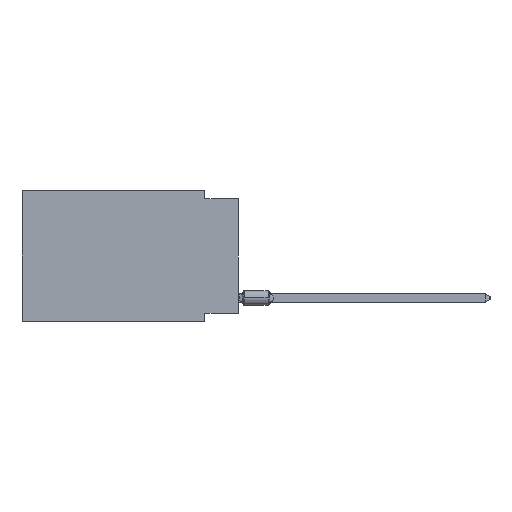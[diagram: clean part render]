
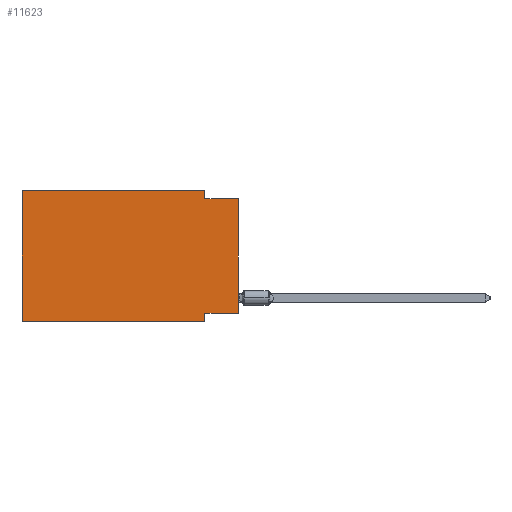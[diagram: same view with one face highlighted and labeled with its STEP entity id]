
A CAD part, left-side view. The second image highlights one B-rep face of the part: STEP entity #11623.
In plain terms, the highlighted planar face has unit normal (-1, 0, 0).
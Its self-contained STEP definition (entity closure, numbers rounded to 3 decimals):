
#2127 = ORIENTED_EDGE ( 'NONE', *, *, #6543, .F. ) ;
#3464 = DIRECTION ( 'NONE',  ( 0., 1., 0. ) ) ;
#3472 = CARTESIAN_POINT ( 'NONE',  ( 0., 16.383, 0. ) ) ;
#4175 = VERTEX_POINT ( 'NONE', #12808 ) ;
#4230 = AXIS2_PLACEMENT_3D ( 'NONE', #32441, #40569, #13186 ) ;
#4279 = CARTESIAN_POINT ( 'NONE',  ( 0., 0., -0.635 ) ) ;
#6543 = EDGE_CURVE ( 'NONE', #8963, #40921, #46497, .T. ) ;
#6654 = CARTESIAN_POINT ( 'NONE',  ( 0., 2.54, 0. ) ) ;
#7289 = FACE_OUTER_BOUND ( 'NONE', #38947, .T. ) ;
#7814 = LINE ( 'NONE', #19885, #52839 ) ;
#8609 = CARTESIAN_POINT ( 'NONE',  ( 0., 2.54, -9.906 ) ) ;
#8963 = VERTEX_POINT ( 'NONE', #3472 ) ;
#9063 = DIRECTION ( 'NONE',  ( 0., -1., 0. ) ) ;
#9440 = CARTESIAN_POINT ( 'NONE',  ( 0., 2.54, 0. ) ) ;
#11123 = EDGE_CURVE ( 'NONE', #50821, #14941, #45249, .T. ) ;
#11400 = ORIENTED_EDGE ( 'NONE', *, *, #36740, .F. ) ;
#11623 = ADVANCED_FACE ( 'NONE', ( #7289 ), #23984, .F. ) ;
#12808 = CARTESIAN_POINT ( 'NONE',  ( 0., 0., -9.271 ) ) ;
#12912 = CARTESIAN_POINT ( 'NONE',  ( 0., 2.54, -9.271 ) ) ;
#13160 = ORIENTED_EDGE ( 'NONE', *, *, #14902, .F. ) ;
#13186 = DIRECTION ( 'NONE',  ( 0., 0., -1. ) ) ;
#14327 = ORIENTED_EDGE ( 'NONE', *, *, #11123, .T. ) ;
#14512 = DIRECTION ( 'NONE',  ( 0., 0., 1. ) ) ;
#14764 = EDGE_CURVE ( 'NONE', #4175, #41214, #7814, .T. ) ;
#14902 = EDGE_CURVE ( 'NONE', #41214, #14941, #46501, .T. ) ;
#14941 = VERTEX_POINT ( 'NONE', #42418 ) ;
#15853 = DIRECTION ( 'NONE',  ( 0., -1., 0. ) ) ;
#16127 = CARTESIAN_POINT ( 'NONE',  ( 0., 16.383, -9.906 ) ) ;
#18914 = ORIENTED_EDGE ( 'NONE', *, *, #36125, .T. ) ;
#19885 = CARTESIAN_POINT ( 'NONE',  ( 0., 0., -9.271 ) ) ;
#21715 = LINE ( 'NONE', #27101, #26157 ) ;
#22663 = EDGE_CURVE ( 'NONE', #50821, #8963, #21715, .T. ) ;
#23984 = PLANE ( 'NONE',  #4230 ) ;
#24459 = ORIENTED_EDGE ( 'NONE', *, *, #47838, .F. ) ;
#26075 = VECTOR ( 'NONE', #14512, 1000. ) ;
#26157 = VECTOR ( 'NONE', #38319, 1000. ) ;
#27101 = CARTESIAN_POINT ( 'NONE',  ( 0., 16.383, 0. ) ) ;
#27835 = VECTOR ( 'NONE', #50324, 1000. ) ;
#29132 = CARTESIAN_POINT ( 'NONE',  ( 0., 16.383, 0. ) ) ;
#29450 = VERTEX_POINT ( 'NONE', #4279 ) ;
#32114 = VECTOR ( 'NONE', #15853, 1000. ) ;
#32441 = CARTESIAN_POINT ( 'NONE',  ( 0., 16.383, 0. ) ) ;
#33035 = CARTESIAN_POINT ( 'NONE',  ( 0., 16.383, -9.906 ) ) ;
#34456 = CARTESIAN_POINT ( 'NONE',  ( 0., 0., -0.635 ) ) ;
#34915 = VECTOR ( 'NONE', #9063, 1000. ) ;
#35318 = ORIENTED_EDGE ( 'NONE', *, *, #22663, .F. ) ;
#36125 = EDGE_CURVE ( 'NONE', #4175, #29450, #48008, .T. ) ;
#36390 = VECTOR ( 'NONE', #38346, 1000. ) ;
#36740 = EDGE_CURVE ( 'NONE', #40921, #49555, #46789, .T. ) ;
#38277 = ORIENTED_EDGE ( 'NONE', *, *, #14764, .F. ) ;
#38319 = DIRECTION ( 'NONE',  ( 0., 0., 1. ) ) ;
#38346 = DIRECTION ( 'NONE',  ( 0., 0., -1. ) ) ;
#38730 = VECTOR ( 'NONE', #45961, 1000. ) ;
#38947 = EDGE_LOOP ( 'NONE', ( #18914, #24459, #11400, #2127, #35318, #14327, #13160, #38277 ) ) ;
#40114 = CARTESIAN_POINT ( 'NONE',  ( 0., 0., 0. ) ) ;
#40569 = DIRECTION ( 'NONE',  ( 1., 0., 0. ) ) ;
#40921 = VERTEX_POINT ( 'NONE', #6654 ) ;
#41214 = VERTEX_POINT ( 'NONE', #12912 ) ;
#42418 = CARTESIAN_POINT ( 'NONE',  ( 0., 2.54, -9.906 ) ) ;
#45249 = LINE ( 'NONE', #16127, #32114 ) ;
#45961 = DIRECTION ( 'NONE',  ( 0., -1., 0. ) ) ;
#46419 = LINE ( 'NONE', #34456, #34915 ) ;
#46497 = LINE ( 'NONE', #29132, #38730 ) ;
#46501 = LINE ( 'NONE', #8609, #36390 ) ;
#46789 = LINE ( 'NONE', #9440, #27835 ) ;
#47155 = CARTESIAN_POINT ( 'NONE',  ( 0., 2.54, -0.635 ) ) ;
#47838 = EDGE_CURVE ( 'NONE', #49555, #29450, #46419, .T. ) ;
#48008 = LINE ( 'NONE', #40114, #26075 ) ;
#49555 = VERTEX_POINT ( 'NONE', #47155 ) ;
#50324 = DIRECTION ( 'NONE',  ( 0., 0., -1. ) ) ;
#50821 = VERTEX_POINT ( 'NONE', #33035 ) ;
#52839 = VECTOR ( 'NONE', #3464, 1000. ) ;
